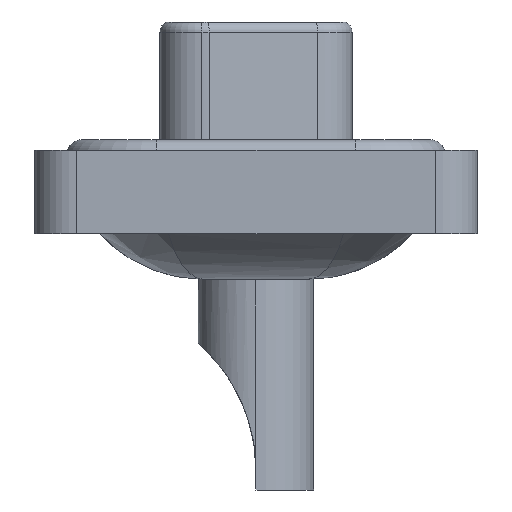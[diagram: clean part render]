
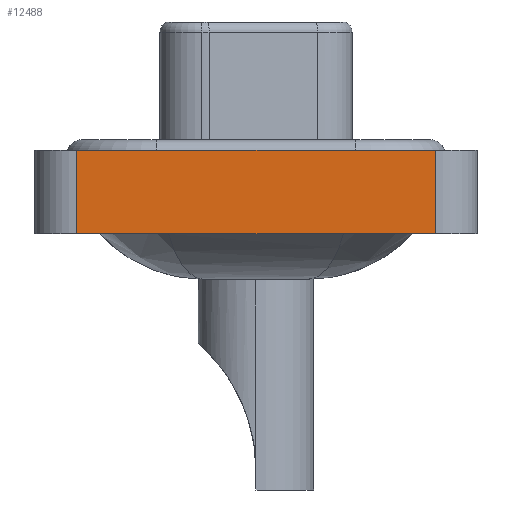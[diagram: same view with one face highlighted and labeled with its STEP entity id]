
A CAD part, left-side view. The second image highlights one B-rep face of the part: STEP entity #12488.
In plain terms, the highlighted planar face has unit normal (-1, 0, 0).
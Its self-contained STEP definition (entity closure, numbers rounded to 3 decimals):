
#514 = EDGE_CURVE ( 'NONE', #2560, #3795, #4685, .T. ) ;
#1628 = DIRECTION ( 'NONE',  ( 0., 0., 1. ) ) ;
#2560 = VERTEX_POINT ( 'NONE', #14040 ) ;
#3359 = DIRECTION ( 'NONE',  ( 0., -1., 0. ) ) ;
#3389 = EDGE_LOOP ( 'NONE', ( #10261, #11426, #12020, #13204 ) ) ;
#3391 = CARTESIAN_POINT ( 'NONE',  ( -7.25, -8.55, 0.4 ) ) ;
#3399 = AXIS2_PLACEMENT_3D ( 'NONE', #6652, #14098, #1628 ) ;
#3795 = VERTEX_POINT ( 'NONE', #3391 ) ;
#3825 = DIRECTION ( 'NONE',  ( 0., 0., 1. ) ) ;
#4685 = LINE ( 'NONE', #10445, #7853 ) ;
#5030 = LINE ( 'NONE', #12193, #5124 ) ;
#5124 = VECTOR ( 'NONE', #16371, 1000. ) ;
#5211 = CARTESIAN_POINT ( 'NONE',  ( -7.25, 8.55, -3.6 ) ) ;
#6318 = VECTOR ( 'NONE', #3825, 1000. ) ;
#6652 = CARTESIAN_POINT ( 'NONE',  ( -7.25, -8.55, -3.6 ) ) ;
#7635 = CARTESIAN_POINT ( 'NONE',  ( -7.25, -8.55, -3.6 ) ) ;
#7790 = VERTEX_POINT ( 'NONE', #14517 ) ;
#7853 = VECTOR ( 'NONE', #16110, 1000. ) ;
#8725 = CARTESIAN_POINT ( 'NONE',  ( -7.25, -8.55, -3.6 ) ) ;
#9596 = VECTOR ( 'NONE', #3359, 1000. ) ;
#9957 = EDGE_CURVE ( 'NONE', #12170, #3795, #5030, .T. ) ;
#9980 = EDGE_CURVE ( 'NONE', #7790, #2560, #12474, .T. ) ;
#10261 = ORIENTED_EDGE ( 'NONE', *, *, #9957, .T. ) ;
#10445 = CARTESIAN_POINT ( 'NONE',  ( -7.25, -8.55, 0.4 ) ) ;
#11426 = ORIENTED_EDGE ( 'NONE', *, *, #514, .F. ) ;
#11794 = EDGE_CURVE ( 'NONE', #7790, #12170, #14960, .T. ) ;
#12020 = ORIENTED_EDGE ( 'NONE', *, *, #9980, .F. ) ;
#12170 = VERTEX_POINT ( 'NONE', #8725 ) ;
#12193 = CARTESIAN_POINT ( 'NONE',  ( -7.25, -8.55, -3.6 ) ) ;
#12474 = LINE ( 'NONE', #5211, #6318 ) ;
#12488 = ADVANCED_FACE ( 'NONE', ( #15128 ), #15404, .T. ) ;
#13204 = ORIENTED_EDGE ( 'NONE', *, *, #11794, .T. ) ;
#14040 = CARTESIAN_POINT ( 'NONE',  ( -7.25, 8.55, 0.4 ) ) ;
#14098 = DIRECTION ( 'NONE',  ( -1., 0., 0. ) ) ;
#14517 = CARTESIAN_POINT ( 'NONE',  ( -7.25, 8.55, -3.6 ) ) ;
#14960 = LINE ( 'NONE', #7635, #9596 ) ;
#15128 = FACE_OUTER_BOUND ( 'NONE', #3389, .T. ) ;
#15404 = PLANE ( 'NONE',  #3399 ) ;
#16110 = DIRECTION ( 'NONE',  ( 0., -1., 0. ) ) ;
#16371 = DIRECTION ( 'NONE',  ( 0., 0., 1. ) ) ;
